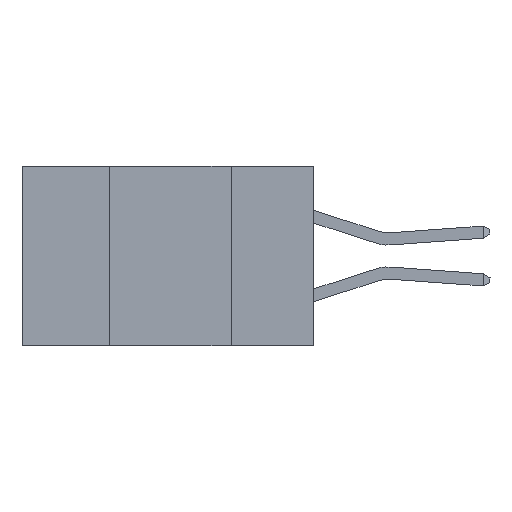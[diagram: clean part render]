
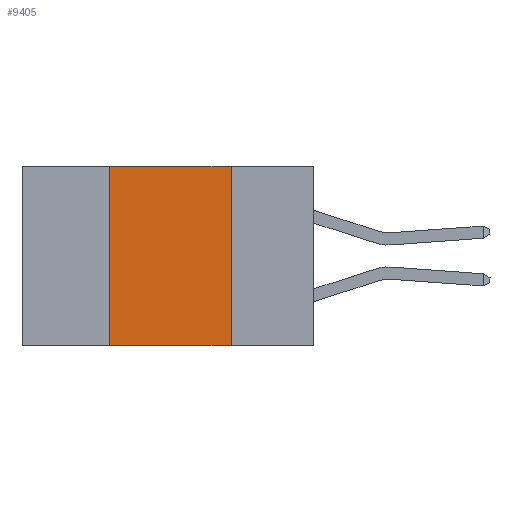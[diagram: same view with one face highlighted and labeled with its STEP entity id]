
A CAD part, left-side view. The second image highlights one B-rep face of the part: STEP entity #9405.
In plain terms, the highlighted planar face has unit normal (-1, 0, 0).
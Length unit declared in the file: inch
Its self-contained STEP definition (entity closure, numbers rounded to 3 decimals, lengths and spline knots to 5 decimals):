
#397 = CARTESIAN_POINT ( 'NONE',  ( 0., 0.17, 0. ) ) ;
#1114 = CARTESIAN_POINT ( 'NONE',  ( 0., 0.17, -0.37 ) ) ;
#1541 = EDGE_CURVE ( 'NONE', #15106, #2532, #8793, .T. ) ;
#1801 = VECTOR ( 'NONE', #6226, 39.37008 ) ;
#2532 = VERTEX_POINT ( 'NONE', #1114 ) ;
#2793 = PLANE ( 'NONE',  #8348 ) ;
#4059 = VECTOR ( 'NONE', #18425, 39.37008 ) ;
#4421 = CARTESIAN_POINT ( 'NONE',  ( 0., 0.6, -0.37 ) ) ;
#4433 = LINE ( 'NONE', #9222, #22462 ) ;
#5623 = DIRECTION ( 'NONE',  ( 0., 0., 1. ) ) ;
#5636 = EDGE_LOOP ( 'NONE', ( #11582, #15130, #14783, #16865 ) ) ;
#6073 = FACE_OUTER_BOUND ( 'NONE', #5636, .T. ) ;
#6226 = DIRECTION ( 'NONE',  ( 0., -1., 0. ) ) ;
#7059 = LINE ( 'NONE', #4421, #1801 ) ;
#7926 = EDGE_CURVE ( 'NONE', #15557, #10840, #4433, .T. ) ;
#8128 = DIRECTION ( 'NONE',  ( 0., 0., -1. ) ) ;
#8348 = AXIS2_PLACEMENT_3D ( 'NONE', #15197, #18662, #8128 ) ;
#8793 = LINE ( 'NONE', #18546, #4059 ) ;
#9222 = CARTESIAN_POINT ( 'NONE',  ( 0., 0.42, 0. ) ) ;
#9405 = ADVANCED_FACE ( 'NONE', ( #6073 ), #2793, .F. ) ;
#10256 = CARTESIAN_POINT ( 'NONE',  ( 0., 0.42, 0. ) ) ;
#10840 = VERTEX_POINT ( 'NONE', #10256 ) ;
#11582 = ORIENTED_EDGE ( 'NONE', *, *, #1541, .F. ) ;
#14783 = ORIENTED_EDGE ( 'NONE', *, *, #7926, .F. ) ;
#15106 = VERTEX_POINT ( 'NONE', #397 ) ;
#15130 = ORIENTED_EDGE ( 'NONE', *, *, #22185, .F. ) ;
#15197 = CARTESIAN_POINT ( 'NONE',  ( 0., 0.6, 0. ) ) ;
#15325 = CARTESIAN_POINT ( 'NONE',  ( 0., 0.6, 0. ) ) ;
#15557 = VERTEX_POINT ( 'NONE', #20922 ) ;
#16865 = ORIENTED_EDGE ( 'NONE', *, *, #17610, .T. ) ;
#17610 = EDGE_CURVE ( 'NONE', #15557, #2532, #7059, .T. ) ;
#18425 = DIRECTION ( 'NONE',  ( 0., 0., -1. ) ) ;
#18546 = CARTESIAN_POINT ( 'NONE',  ( 0., 0.17, 0. ) ) ;
#18662 = DIRECTION ( 'NONE',  ( 1., 0., 0. ) ) ;
#18789 = DIRECTION ( 'NONE',  ( 0., -1., 0. ) ) ;
#20922 = CARTESIAN_POINT ( 'NONE',  ( 0., 0.42, -0.37 ) ) ;
#21865 = VECTOR ( 'NONE', #18789, 39.37008 ) ;
#22185 = EDGE_CURVE ( 'NONE', #10840, #15106, #22369, .T. ) ;
#22369 = LINE ( 'NONE', #15325, #21865 ) ;
#22462 = VECTOR ( 'NONE', #5623, 39.37008 ) ;
